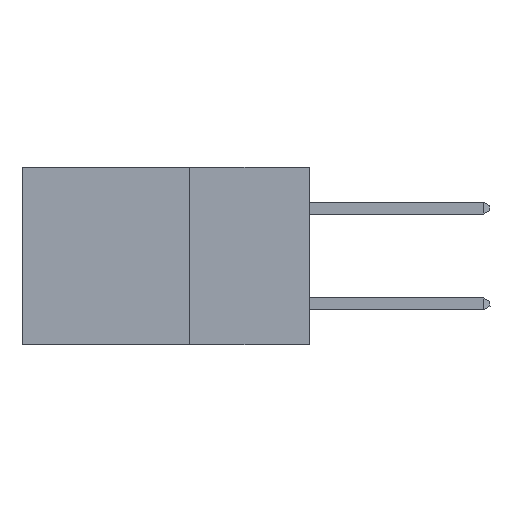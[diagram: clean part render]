
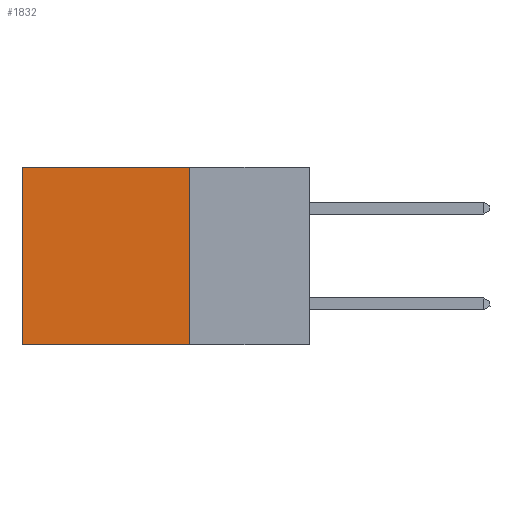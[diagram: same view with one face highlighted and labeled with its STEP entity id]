
A CAD part, left-side view. The second image highlights one B-rep face of the part: STEP entity #1832.
In plain terms, the highlighted planar face has unit normal (-1, 0, 0).
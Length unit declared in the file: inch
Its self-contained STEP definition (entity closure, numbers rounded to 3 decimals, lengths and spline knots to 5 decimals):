
#294 = EDGE_LOOP ( 'NONE', ( #7584, #808, #5723, #4207 ) ) ;
#340 = CARTESIAN_POINT ( 'NONE',  ( 0.2875, 0.25, -0.37 ) ) ;
#808 = ORIENTED_EDGE ( 'NONE', *, *, #11182, .F. ) ;
#1534 = DIRECTION ( 'NONE',  ( 0., 1., 0. ) ) ;
#1832 = ADVANCED_FACE ( 'NONE', ( #5417 ), #3188, .F. ) ;
#2860 = CARTESIAN_POINT ( 'NONE',  ( 0.2875, 0.25, 0. ) ) ;
#3096 = AXIS2_PLACEMENT_3D ( 'NONE', #8607, #10422, #22845 ) ;
#3188 = PLANE ( 'NONE',  #3096 ) ;
#4207 = ORIENTED_EDGE ( 'NONE', *, *, #18662, .T. ) ;
#4275 = VECTOR ( 'NONE', #1534, 39.37008 ) ;
#5417 = FACE_OUTER_BOUND ( 'NONE', #294, .T. ) ;
#5723 = ORIENTED_EDGE ( 'NONE', *, *, #12965, .F. ) ;
#6192 = VECTOR ( 'NONE', #10441, 39.37008 ) ;
#6739 = LINE ( 'NONE', #340, #17871 ) ;
#7584 = ORIENTED_EDGE ( 'NONE', *, *, #19684, .T. ) ;
#8607 = CARTESIAN_POINT ( 'NONE',  ( 0.2875, 0.25, 0. ) ) ;
#10021 = DIRECTION ( 'NONE',  ( 0., 0., -1. ) ) ;
#10185 = LINE ( 'NONE', #14014, #4275 ) ;
#10422 = DIRECTION ( 'NONE',  ( 1., 0., 0. ) ) ;
#10441 = DIRECTION ( 'NONE',  ( 0., 0., -1. ) ) ;
#11182 = EDGE_CURVE ( 'NONE', #22391, #17277, #6739, .T. ) ;
#12965 = EDGE_CURVE ( 'NONE', #21978, #22391, #19997, .T. ) ;
#14014 = CARTESIAN_POINT ( 'NONE',  ( 0.2875, 0.25, 0. ) ) ;
#14222 = CARTESIAN_POINT ( 'NONE',  ( 0.2875, 0.6, -0.37 ) ) ;
#14677 = DIRECTION ( 'NONE',  ( 0., 1., 0. ) ) ;
#15814 = VECTOR ( 'NONE', #10021, 39.37008 ) ;
#17262 = CARTESIAN_POINT ( 'NONE',  ( 0.2875, 0.6, 0. ) ) ;
#17277 = VERTEX_POINT ( 'NONE', #14222 ) ;
#17871 = VECTOR ( 'NONE', #14677, 39.37008 ) ;
#18662 = EDGE_CURVE ( 'NONE', #21978, #22316, #10185, .T. ) ;
#19684 = EDGE_CURVE ( 'NONE', #22316, #17277, #19862, .T. ) ;
#19862 = LINE ( 'NONE', #21078, #6192 ) ;
#19927 = CARTESIAN_POINT ( 'NONE',  ( 0.2875, 0.25, 0. ) ) ;
#19997 = LINE ( 'NONE', #2860, #15814 ) ;
#21078 = CARTESIAN_POINT ( 'NONE',  ( 0.2875, 0.6, 0. ) ) ;
#21978 = VERTEX_POINT ( 'NONE', #19927 ) ;
#22316 = VERTEX_POINT ( 'NONE', #17262 ) ;
#22391 = VERTEX_POINT ( 'NONE', #22932 ) ;
#22845 = DIRECTION ( 'NONE',  ( 0., 0., -1. ) ) ;
#22932 = CARTESIAN_POINT ( 'NONE',  ( 0.2875, 0.25, -0.37 ) ) ;
